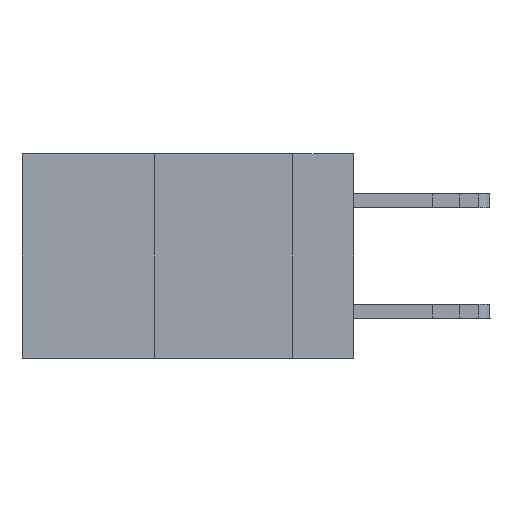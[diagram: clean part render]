
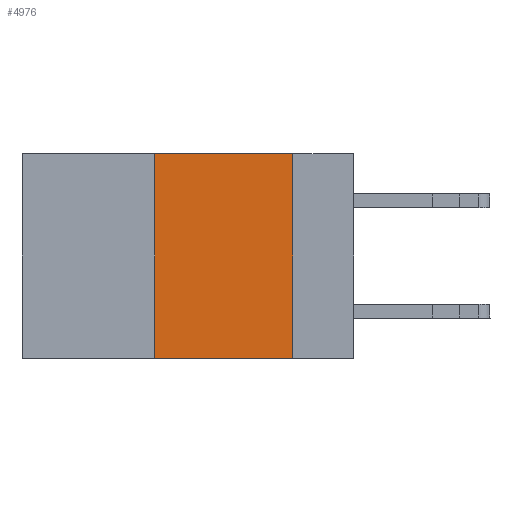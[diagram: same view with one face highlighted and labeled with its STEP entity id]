
A CAD part, left-side view. The second image highlights one B-rep face of the part: STEP entity #4976.
In plain terms, the highlighted planar face has unit normal (-1, 0, 0).
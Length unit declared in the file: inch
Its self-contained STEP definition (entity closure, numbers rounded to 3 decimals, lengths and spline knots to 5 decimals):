
#876 = CARTESIAN_POINT ( 'NONE',  ( 0., 0.36, -0.37 ) ) ;
#963 = CARTESIAN_POINT ( 'NONE',  ( 0., 0.11, 0. ) ) ;
#1633 = LINE ( 'NONE', #963, #9011 ) ;
#2518 = DIRECTION ( 'NONE',  ( 0., 0., -1. ) ) ;
#2706 = CARTESIAN_POINT ( 'NONE',  ( 0., 0.36, 0. ) ) ;
#3106 = DIRECTION ( 'NONE',  ( 0., 0., 1. ) ) ;
#3872 = DIRECTION ( 'NONE',  ( 0., -1., 0. ) ) ;
#4976 = ADVANCED_FACE ( 'NONE', ( #10621 ), #12566, .F. ) ;
#5063 = CARTESIAN_POINT ( 'NONE',  ( 0., 0.11, 0. ) ) ;
#6627 = CARTESIAN_POINT ( 'NONE',  ( 0., 0.6, -0.37 ) ) ;
#6920 = DIRECTION ( 'NONE',  ( 1., 0., 0. ) ) ;
#6934 = EDGE_CURVE ( 'NONE', #17076, #12884, #1633, .T. ) ;
#7127 = VECTOR ( 'NONE', #3872, 39.37008 ) ;
#7460 = ORIENTED_EDGE ( 'NONE', *, *, #17502, .F. ) ;
#7527 = VECTOR ( 'NONE', #3106, 39.37008 ) ;
#8095 = VERTEX_POINT ( 'NONE', #876 ) ;
#8783 = VECTOR ( 'NONE', #16679, 39.37008 ) ;
#8802 = CARTESIAN_POINT ( 'NONE',  ( 0., 0.6, 0. ) ) ;
#9011 = VECTOR ( 'NONE', #2518, 39.37008 ) ;
#10621 = FACE_OUTER_BOUND ( 'NONE', #11974, .T. ) ;
#10840 = ORIENTED_EDGE ( 'NONE', *, *, #15994, .F. ) ;
#11136 = CARTESIAN_POINT ( 'NONE',  ( 0., 0.6, 0. ) ) ;
#11752 = ORIENTED_EDGE ( 'NONE', *, *, #13993, .T. ) ;
#11974 = EDGE_LOOP ( 'NONE', ( #14218, #10840, #7460, #11752 ) ) ;
#12566 = PLANE ( 'NONE',  #13420 ) ;
#12884 = VERTEX_POINT ( 'NONE', #17088 ) ;
#13420 = AXIS2_PLACEMENT_3D ( 'NONE', #8802, #6920, #15643 ) ;
#13993 = EDGE_CURVE ( 'NONE', #8095, #12884, #16380, .T. ) ;
#14218 = ORIENTED_EDGE ( 'NONE', *, *, #6934, .F. ) ;
#15643 = DIRECTION ( 'NONE',  ( 0., 0., -1. ) ) ;
#15994 = EDGE_CURVE ( 'NONE', #16643, #17076, #18070, .T. ) ;
#16380 = LINE ( 'NONE', #6627, #8783 ) ;
#16643 = VERTEX_POINT ( 'NONE', #2706 ) ;
#16679 = DIRECTION ( 'NONE',  ( 0., -1., 0. ) ) ;
#17076 = VERTEX_POINT ( 'NONE', #5063 ) ;
#17088 = CARTESIAN_POINT ( 'NONE',  ( 0., 0.11, -0.37 ) ) ;
#17502 = EDGE_CURVE ( 'NONE', #8095, #16643, #18467, .T. ) ;
#17513 = CARTESIAN_POINT ( 'NONE',  ( 0., 0.36, 0. ) ) ;
#18070 = LINE ( 'NONE', #11136, #7127 ) ;
#18467 = LINE ( 'NONE', #17513, #7527 ) ;
